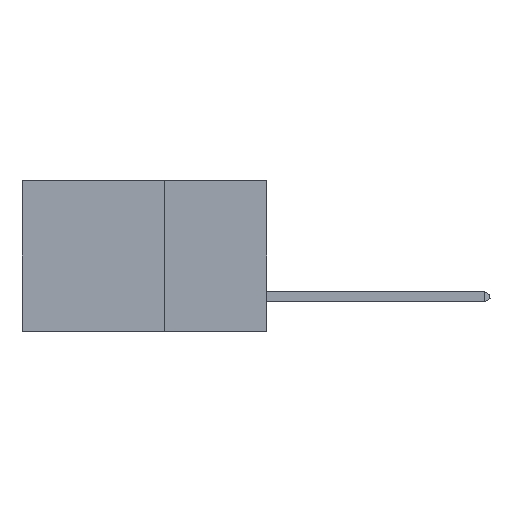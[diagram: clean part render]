
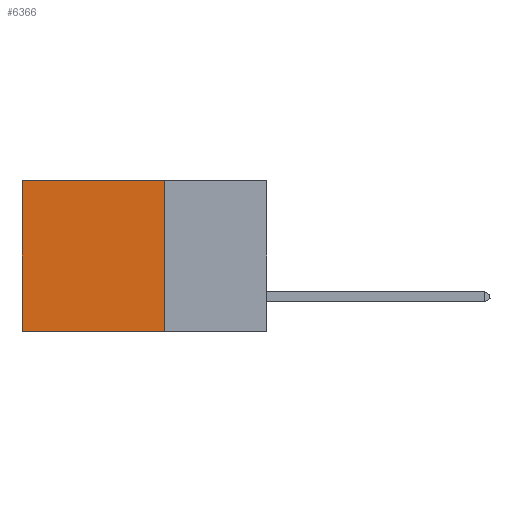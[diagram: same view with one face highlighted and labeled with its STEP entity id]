
A CAD part, left-side view. The second image highlights one B-rep face of the part: STEP entity #6366.
In plain terms, the highlighted planar face has unit normal (-1, 0, 0).
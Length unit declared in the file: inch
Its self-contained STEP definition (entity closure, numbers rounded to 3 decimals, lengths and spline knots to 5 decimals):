
#1020 = DIRECTION ( 'NONE',  ( 0., 1., 0. ) ) ;
#1676 = CARTESIAN_POINT ( 'NONE',  ( 0.2875, 0.25, 0. ) ) ;
#3309 = CARTESIAN_POINT ( 'NONE',  ( 0.2875, 0.6, 0. ) ) ;
#3723 = CARTESIAN_POINT ( 'NONE',  ( 0.2875, 0.6, 0. ) ) ;
#3874 = CARTESIAN_POINT ( 'NONE',  ( 0.2875, 0.6, -0.37 ) ) ;
#3881 = DIRECTION ( 'NONE',  ( 0., 0., -1. ) ) ;
#4939 = EDGE_CURVE ( 'NONE', #22119, #20357, #15039, .T. ) ;
#6169 = ORIENTED_EDGE ( 'NONE', *, *, #18837, .F. ) ;
#6366 = ADVANCED_FACE ( 'NONE', ( #18376 ), #18565, .F. ) ;
#6435 = DIRECTION ( 'NONE',  ( 0., 0., -1. ) ) ;
#7051 = CARTESIAN_POINT ( 'NONE',  ( 0.2875, 0.25, -0.37 ) ) ;
#7152 = EDGE_CURVE ( 'NONE', #22119, #18124, #17797, .T. ) ;
#7668 = VECTOR ( 'NONE', #20258, 39.37008 ) ;
#8091 = VECTOR ( 'NONE', #1020, 39.37008 ) ;
#8549 = CARTESIAN_POINT ( 'NONE',  ( 0.2875, 0.25, 0. ) ) ;
#9040 = CARTESIAN_POINT ( 'NONE',  ( 0.2875, 0.25, -0.37 ) ) ;
#9224 = ORIENTED_EDGE ( 'NONE', *, *, #20449, .T. ) ;
#9491 = CARTESIAN_POINT ( 'NONE',  ( 0.2875, 0.25, 0. ) ) ;
#9988 = LINE ( 'NONE', #7051, #7668 ) ;
#11353 = VECTOR ( 'NONE', #3881, 39.37008 ) ;
#11655 = DIRECTION ( 'NONE',  ( 1., 0., 0. ) ) ;
#15039 = LINE ( 'NONE', #19273, #21558 ) ;
#15253 = DIRECTION ( 'NONE',  ( 0., 0., -1. ) ) ;
#16219 = LINE ( 'NONE', #3723, #11353 ) ;
#16434 = ORIENTED_EDGE ( 'NONE', *, *, #7152, .T. ) ;
#17129 = EDGE_LOOP ( 'NONE', ( #9224, #6169, #23563, #16434 ) ) ;
#17658 = VERTEX_POINT ( 'NONE', #3874 ) ;
#17797 = LINE ( 'NONE', #8549, #8091 ) ;
#18124 = VERTEX_POINT ( 'NONE', #3309 ) ;
#18376 = FACE_OUTER_BOUND ( 'NONE', #17129, .T. ) ;
#18565 = PLANE ( 'NONE',  #20169 ) ;
#18837 = EDGE_CURVE ( 'NONE', #20357, #17658, #9988, .T. ) ;
#19273 = CARTESIAN_POINT ( 'NONE',  ( 0.2875, 0.25, 0. ) ) ;
#20169 = AXIS2_PLACEMENT_3D ( 'NONE', #9491, #11655, #15253 ) ;
#20258 = DIRECTION ( 'NONE',  ( 0., 1., 0. ) ) ;
#20357 = VERTEX_POINT ( 'NONE', #9040 ) ;
#20449 = EDGE_CURVE ( 'NONE', #18124, #17658, #16219, .T. ) ;
#21558 = VECTOR ( 'NONE', #6435, 39.37008 ) ;
#22119 = VERTEX_POINT ( 'NONE', #1676 ) ;
#23563 = ORIENTED_EDGE ( 'NONE', *, *, #4939, .F. ) ;
